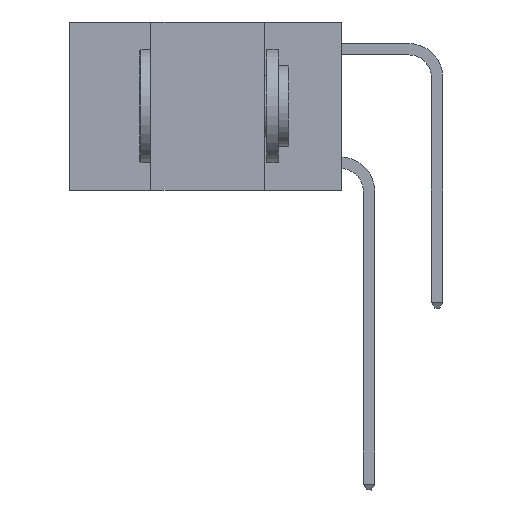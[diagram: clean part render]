
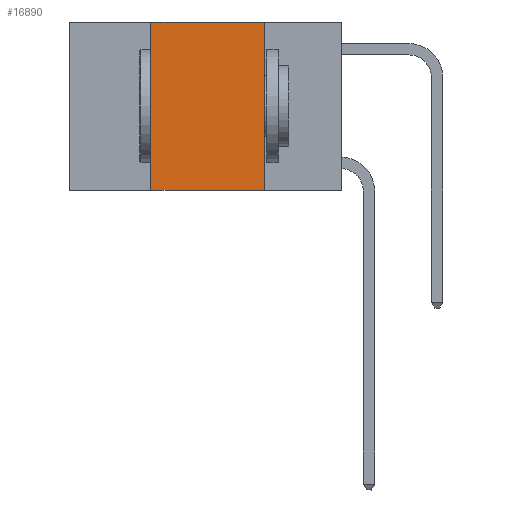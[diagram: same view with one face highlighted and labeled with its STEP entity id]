
A CAD part, left-side view. The second image highlights one B-rep face of the part: STEP entity #16890.
In plain terms, the highlighted planar face has unit normal (-1, 0, 0).
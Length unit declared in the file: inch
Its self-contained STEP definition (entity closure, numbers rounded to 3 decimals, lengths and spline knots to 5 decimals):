
#418 = CARTESIAN_POINT ( 'NONE',  ( 0., 0.42, -0.37 ) ) ;
#513 = VECTOR ( 'NONE', #4120, 39.37008 ) ;
#519 = CARTESIAN_POINT ( 'NONE',  ( 0., 0.6, -0.37 ) ) ;
#764 = CARTESIAN_POINT ( 'NONE',  ( 0., 0.42, 0. ) ) ;
#1598 = ORIENTED_EDGE ( 'NONE', *, *, #4068, .F. ) ;
#2068 = LINE ( 'NONE', #764, #10860 ) ;
#3814 = AXIS2_PLACEMENT_3D ( 'NONE', #11951, #6126, #18055 ) ;
#3840 = CARTESIAN_POINT ( 'NONE',  ( 0., 0.17, 0. ) ) ;
#4068 = EDGE_CURVE ( 'NONE', #12809, #10901, #2068, .T. ) ;
#4120 = DIRECTION ( 'NONE',  ( 0., -1., 0. ) ) ;
#5384 = CARTESIAN_POINT ( 'NONE',  ( 0., 0.17, -0.37 ) ) ;
#6126 = DIRECTION ( 'NONE',  ( 1., 0., 0. ) ) ;
#6153 = VECTOR ( 'NONE', #8882, 39.37008 ) ;
#6909 = EDGE_LOOP ( 'NONE', ( #7474, #10096, #1598, #15826 ) ) ;
#7075 = VECTOR ( 'NONE', #10867, 39.37008 ) ;
#7474 = ORIENTED_EDGE ( 'NONE', *, *, #17560, .F. ) ;
#7623 = PLANE ( 'NONE',  #3814 ) ;
#7991 = LINE ( 'NONE', #14681, #6153 ) ;
#8017 = CARTESIAN_POINT ( 'NONE',  ( 0., 0.42, 0. ) ) ;
#8882 = DIRECTION ( 'NONE',  ( 0., 0., -1. ) ) ;
#10096 = ORIENTED_EDGE ( 'NONE', *, *, #15027, .F. ) ;
#10168 = VERTEX_POINT ( 'NONE', #3840 ) ;
#10860 = VECTOR ( 'NONE', #11111, 39.37008 ) ;
#10867 = DIRECTION ( 'NONE',  ( 0., -1., 0. ) ) ;
#10901 = VERTEX_POINT ( 'NONE', #8017 ) ;
#11111 = DIRECTION ( 'NONE',  ( 0., 0., 1. ) ) ;
#11951 = CARTESIAN_POINT ( 'NONE',  ( 0., 0.6, 0. ) ) ;
#12809 = VERTEX_POINT ( 'NONE', #418 ) ;
#12936 = CARTESIAN_POINT ( 'NONE',  ( 0., 0.6, 0. ) ) ;
#13426 = LINE ( 'NONE', #519, #7075 ) ;
#14173 = FACE_OUTER_BOUND ( 'NONE', #6909, .T. ) ;
#14573 = EDGE_CURVE ( 'NONE', #12809, #15485, #13426, .T. ) ;
#14681 = CARTESIAN_POINT ( 'NONE',  ( 0., 0.17, 0. ) ) ;
#15027 = EDGE_CURVE ( 'NONE', #10901, #10168, #16184, .T. ) ;
#15485 = VERTEX_POINT ( 'NONE', #5384 ) ;
#15826 = ORIENTED_EDGE ( 'NONE', *, *, #14573, .T. ) ;
#16184 = LINE ( 'NONE', #12936, #513 ) ;
#16890 = ADVANCED_FACE ( 'NONE', ( #14173 ), #7623, .F. ) ;
#17560 = EDGE_CURVE ( 'NONE', #10168, #15485, #7991, .T. ) ;
#18055 = DIRECTION ( 'NONE',  ( 0., 0., -1. ) ) ;
